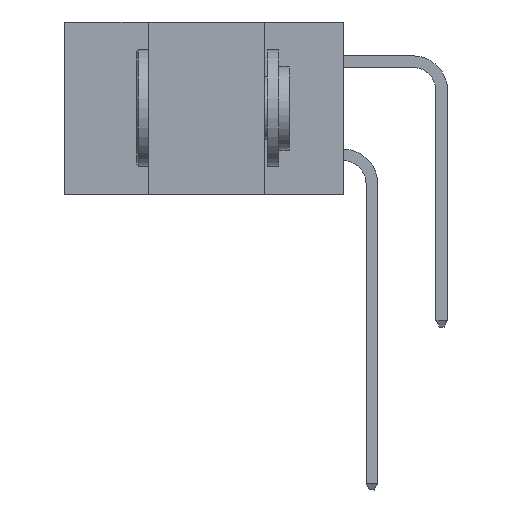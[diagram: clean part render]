
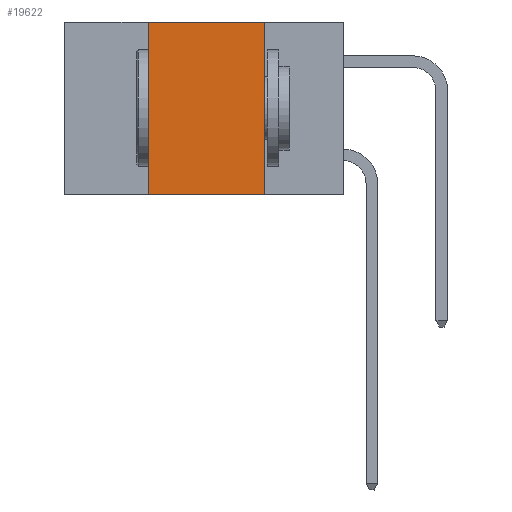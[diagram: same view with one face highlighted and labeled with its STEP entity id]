
A CAD part, left-side view. The second image highlights one B-rep face of the part: STEP entity #19622.
In plain terms, the highlighted planar face has unit normal (-1, 0, 0).
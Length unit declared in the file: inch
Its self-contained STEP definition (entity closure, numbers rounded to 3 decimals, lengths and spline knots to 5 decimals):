
#747 = DIRECTION ( 'NONE',  ( 0., 0., -1. ) ) ;
#2133 = VECTOR ( 'NONE', #23223, 39.37008 ) ;
#2566 = PLANE ( 'NONE',  #15676 ) ;
#2657 = VERTEX_POINT ( 'NONE', #16347 ) ;
#3213 = CARTESIAN_POINT ( 'NONE',  ( 0., 0.17, 0. ) ) ;
#3807 = LINE ( 'NONE', #9226, #8274 ) ;
#5858 = ORIENTED_EDGE ( 'NONE', *, *, #7712, .F. ) ;
#7252 = VECTOR ( 'NONE', #15227, 39.37008 ) ;
#7712 = EDGE_CURVE ( 'NONE', #14161, #9837, #19804, .T. ) ;
#8274 = VECTOR ( 'NONE', #11140, 39.37008 ) ;
#8301 = CARTESIAN_POINT ( 'NONE',  ( 0., 0.6, 0. ) ) ;
#8855 = ORIENTED_EDGE ( 'NONE', *, *, #20414, .F. ) ;
#9226 = CARTESIAN_POINT ( 'NONE',  ( 0., 0.6, 0. ) ) ;
#9791 = ORIENTED_EDGE ( 'NONE', *, *, #17884, .F. ) ;
#9837 = VERTEX_POINT ( 'NONE', #17839 ) ;
#10057 = CARTESIAN_POINT ( 'NONE',  ( 0., 0.6, -0.37 ) ) ;
#11012 = CARTESIAN_POINT ( 'NONE',  ( 0., 0.17, -0.37 ) ) ;
#11140 = DIRECTION ( 'NONE',  ( 0., -1., 0. ) ) ;
#11339 = CARTESIAN_POINT ( 'NONE',  ( 0., 0.42, -0.37 ) ) ;
#11868 = EDGE_CURVE ( 'NONE', #15070, #9837, #22851, .T. ) ;
#12153 = DIRECTION ( 'NONE',  ( 1., 0., 0. ) ) ;
#13312 = CARTESIAN_POINT ( 'NONE',  ( 0., 0.42, -0.37 ) ) ;
#14161 = VERTEX_POINT ( 'NONE', #3213 ) ;
#14821 = VECTOR ( 'NONE', #18605, 39.37008 ) ;
#15070 = VERTEX_POINT ( 'NONE', #11339 ) ;
#15227 = DIRECTION ( 'NONE',  ( 0., 0., 1. ) ) ;
#15676 = AXIS2_PLACEMENT_3D ( 'NONE', #8301, #12153, #747 ) ;
#16347 = CARTESIAN_POINT ( 'NONE',  ( 0., 0.42, 0. ) ) ;
#17673 = EDGE_LOOP ( 'NONE', ( #5858, #9791, #8855, #21302 ) ) ;
#17839 = CARTESIAN_POINT ( 'NONE',  ( 0., 0.17, -0.37 ) ) ;
#17884 = EDGE_CURVE ( 'NONE', #2657, #14161, #3807, .T. ) ;
#18605 = DIRECTION ( 'NONE',  ( 0., 0., -1. ) ) ;
#19622 = ADVANCED_FACE ( 'NONE', ( #23824 ), #2566, .F. ) ;
#19804 = LINE ( 'NONE', #11012, #14821 ) ;
#20414 = EDGE_CURVE ( 'NONE', #15070, #2657, #22336, .T. ) ;
#21302 = ORIENTED_EDGE ( 'NONE', *, *, #11868, .T. ) ;
#22336 = LINE ( 'NONE', #13312, #7252 ) ;
#22851 = LINE ( 'NONE', #10057, #2133 ) ;
#23223 = DIRECTION ( 'NONE',  ( 0., -1., 0. ) ) ;
#23824 = FACE_OUTER_BOUND ( 'NONE', #17673, .T. ) ;
